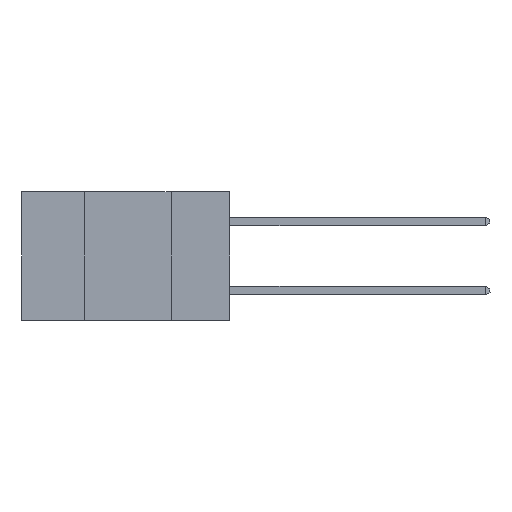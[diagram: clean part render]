
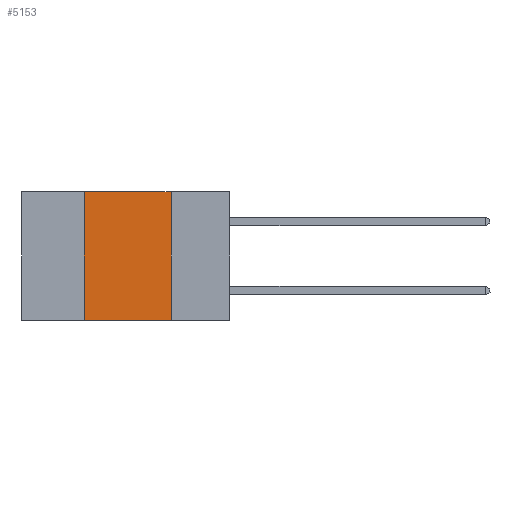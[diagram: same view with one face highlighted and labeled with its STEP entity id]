
A CAD part, left-side view. The second image highlights one B-rep face of the part: STEP entity #5153.
In plain terms, the highlighted planar face has unit normal (-1, 0, 0).
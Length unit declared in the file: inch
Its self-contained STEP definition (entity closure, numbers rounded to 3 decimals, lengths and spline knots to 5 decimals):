
#184 = VERTEX_POINT ( 'NONE', #10881 ) ;
#548 = EDGE_LOOP ( 'NONE', ( #12554, #10973, #10121, #16320 ) ) ;
#1342 = FACE_OUTER_BOUND ( 'NONE', #548, .T. ) ;
#1357 = DIRECTION ( 'NONE',  ( 0., 0., -1. ) ) ;
#1662 = CARTESIAN_POINT ( 'NONE',  ( 0., 0.17, 0. ) ) ;
#2571 = DIRECTION ( 'NONE',  ( 0., -1., 0. ) ) ;
#2971 = CARTESIAN_POINT ( 'NONE',  ( 0., 0.17, 0. ) ) ;
#2976 = VECTOR ( 'NONE', #12756, 39.37008 ) ;
#3269 = EDGE_CURVE ( 'NONE', #7041, #184, #13095, .T. ) ;
#4667 = EDGE_CURVE ( 'NONE', #184, #8935, #13242, .T. ) ;
#4750 = EDGE_CURVE ( 'NONE', #7041, #15764, #9844, .T. ) ;
#5139 = PLANE ( 'NONE',  #10403 ) ;
#5153 = ADVANCED_FACE ( 'NONE', ( #1342 ), #5139, .F. ) ;
#6083 = VECTOR ( 'NONE', #2571, 39.37008 ) ;
#6430 = DIRECTION ( 'NONE',  ( 1., 0., 0. ) ) ;
#7041 = VERTEX_POINT ( 'NONE', #11473 ) ;
#7616 = CARTESIAN_POINT ( 'NONE',  ( 0., 0.42, 0. ) ) ;
#8543 = VECTOR ( 'NONE', #9462, 39.37008 ) ;
#8935 = VERTEX_POINT ( 'NONE', #2971 ) ;
#8948 = LINE ( 'NONE', #1662, #8543 ) ;
#8961 = EDGE_CURVE ( 'NONE', #8935, #15764, #8948, .T. ) ;
#9031 = CARTESIAN_POINT ( 'NONE',  ( 0., 0.6, 0. ) ) ;
#9462 = DIRECTION ( 'NONE',  ( 0., 0., -1. ) ) ;
#9844 = LINE ( 'NONE', #14054, #6083 ) ;
#10121 = ORIENTED_EDGE ( 'NONE', *, *, #3269, .F. ) ;
#10152 = CARTESIAN_POINT ( 'NONE',  ( 0., 0.6, 0. ) ) ;
#10403 = AXIS2_PLACEMENT_3D ( 'NONE', #9031, #6430, #1357 ) ;
#10881 = CARTESIAN_POINT ( 'NONE',  ( 0., 0.42, 0. ) ) ;
#10973 = ORIENTED_EDGE ( 'NONE', *, *, #4667, .F. ) ;
#11473 = CARTESIAN_POINT ( 'NONE',  ( 0., 0.42, -0.37 ) ) ;
#11637 = VECTOR ( 'NONE', #12715, 39.37008 ) ;
#12238 = CARTESIAN_POINT ( 'NONE',  ( 0., 0.17, -0.37 ) ) ;
#12554 = ORIENTED_EDGE ( 'NONE', *, *, #8961, .F. ) ;
#12715 = DIRECTION ( 'NONE',  ( 0., -1., 0. ) ) ;
#12756 = DIRECTION ( 'NONE',  ( 0., 0., 1. ) ) ;
#13095 = LINE ( 'NONE', #7616, #2976 ) ;
#13242 = LINE ( 'NONE', #10152, #11637 ) ;
#14054 = CARTESIAN_POINT ( 'NONE',  ( 0., 0.6, -0.37 ) ) ;
#15764 = VERTEX_POINT ( 'NONE', #12238 ) ;
#16320 = ORIENTED_EDGE ( 'NONE', *, *, #4750, .T. ) ;
